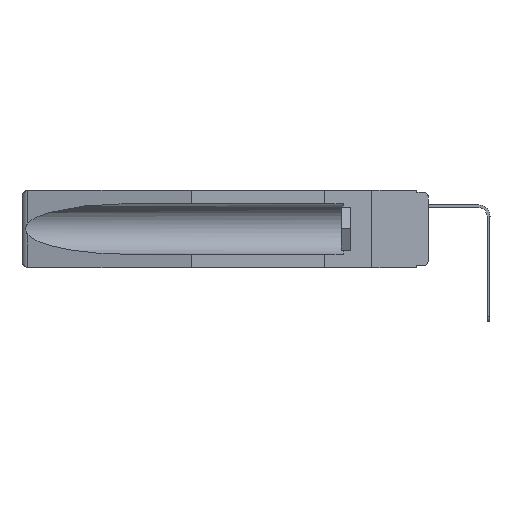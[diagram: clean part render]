
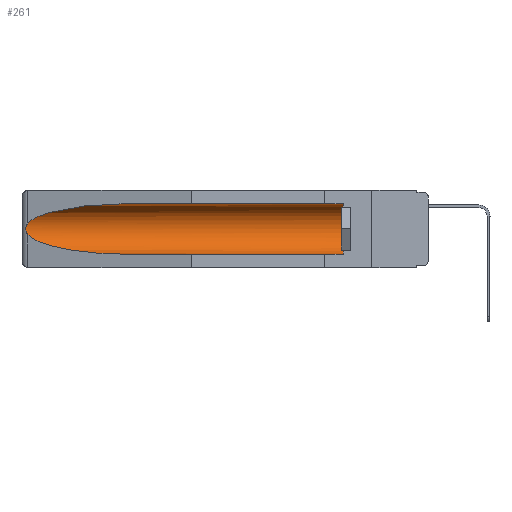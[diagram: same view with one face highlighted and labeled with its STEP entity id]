
A CAD part, left-side view. The second image highlights one B-rep face of the part: STEP entity #261.
In plain terms, the highlighted cylindrical face has radius 2.857 mm (diameter 5.715 mm), a partial arc.
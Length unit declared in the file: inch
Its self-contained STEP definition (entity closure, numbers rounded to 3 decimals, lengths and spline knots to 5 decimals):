
#261 = ADVANCED_FACE ( 'NONE', ( #9949 ), #20373, .F. ) ;
#1026 = DIRECTION ( 'NONE',  ( 0., 1., 0. ) ) ;
#1348 = EDGE_CURVE ( 'NONE', #8231, #16953, #18255, .T. ) ;
#1797 = ORIENTED_EDGE ( 'NONE', *, *, #7680, .F. ) ;
#2048 = CARTESIAN_POINT ( 'NONE',  ( 0.2673, 1.53269, -0.17917 ) ) ;
#2717 = CARTESIAN_POINT ( 'NONE',  ( 0.155, -0.30754, -0.059 ) ) ;
#2866 = DIRECTION ( 'NONE',  ( 0., -1., 0. ) ) ;
#4016 = DIRECTION ( 'NONE',  ( 0., 1., 0. ) ) ;
#4052 = VECTOR ( 'NONE', #4016, 39.37008 ) ;
#4215 = CARTESIAN_POINT ( 'NONE',  ( 0.21114, 1.30732, -0.059 ) ) ;
#4365 = CARTESIAN_POINT ( 'NONE',  ( 0.155, -0.30754, -0.1715 ) ) ;
#4412 = VECTOR ( 'NONE', #20978, 39.37008 ) ;
#4513 = DIRECTION ( 'NONE',  ( 0., 0., 1. ) ) ;
#5088 =( BOUNDED_CURVE ( )  B_SPLINE_CURVE ( 3, ( #14049, #4215, #5891, #16019 ),
 .UNSPECIFIED., .F., .T. ) 
 B_SPLINE_CURVE_WITH_KNOTS ( ( 4, 4 ),
 ( 4.71239, 6.08839 ),
 .UNSPECIFIED. ) 
 CURVE ( )  GEOMETRIC_REPRESENTATION_ITEM ( )  RATIONAL_B_SPLINE_CURVE ( ( 1., 0.848, 0.848, 1. ) ) 
 REPRESENTATION_ITEM ( '' )  );
#5197 = AXIS2_PLACEMENT_3D ( 'NONE', #4365, #1026, #14194 ) ;
#5366 = CARTESIAN_POINT ( 'NONE',  ( 0.26654, 1.53092, -0.15636 ) ) ;
#5609 = EDGE_LOOP ( 'NONE', ( #21602, #20404, #14075, #1797, #11931, #19507 ) ) ;
#5735 = EDGE_CURVE ( 'NONE', #16953, #8511, #5088, .T. ) ;
#5739 = CIRCLE ( 'NONE', #12850, 0.1125 ) ;
#5891 = CARTESIAN_POINT ( 'NONE',  ( 0.25451, 1.48313, -0.09465 ) ) ;
#6715 = CARTESIAN_POINT ( 'NONE',  ( 0.155, 0.126, -0.059 ) ) ;
#6747 = CARTESIAN_POINT ( 'NONE',  ( 0.26655, 1.53094, -0.18657 ) ) ;
#7036 = CARTESIAN_POINT ( 'NONE',  ( 0.2675, 1.53308, -0.16763 ) ) ;
#7680 = EDGE_CURVE ( 'NONE', #8990, #16061, #11639, .T. ) ;
#8231 = VERTEX_POINT ( 'NONE', #6715 ) ;
#8350 = CARTESIAN_POINT ( 'NONE',  ( 0.155, 1.07973, -0.059 ) ) ;
#8511 = VERTEX_POINT ( 'NONE', #13926 ) ;
#8990 = VERTEX_POINT ( 'NONE', #18480 ) ;
#9949 = FACE_OUTER_BOUND ( 'NONE', #5609, .T. ) ;
#10250 = CARTESIAN_POINT ( 'NONE',  ( 0.26597, 1.52961, -0.15275 ) ) ;
#10325 = CARTESIAN_POINT ( 'NONE',  ( 0.26537, 1.52718, -0.14972 ) ) ;
#10452 = CARTESIAN_POINT ( 'NONE',  ( 0.155, 1.07973, -0.284 ) ) ;
#10536 = CARTESIAN_POINT ( 'NONE',  ( 0.25451, 1.48313, -0.24835 ) ) ;
#10671 = CARTESIAN_POINT ( 'NONE',  ( 0.155, -0.30754, -0.284 ) ) ;
#11226 = CARTESIAN_POINT ( 'NONE',  ( 0.155, 0.126, -0.1715 ) ) ;
#11639 = LINE ( 'NONE', #10671, #4052 ) ;
#11931 = ORIENTED_EDGE ( 'NONE', *, *, #16201, .T. ) ;
#12039 = CARTESIAN_POINT ( 'NONE',  ( 0.26537, 1.52718, -0.19328 ) ) ;
#12171 = B_SPLINE_CURVE_WITH_KNOTS ( 'NONE', 3,
 ( #10325, #10250, #5366, #17023, #7036, #18706, #2048, #6747, #18424, #20079 ),
 .UNSPECIFIED., .F., .F.,
 ( 4, 2, 2, 2, 4 ),
 ( 0., 0.00029, 0.00058, 0.00087, 0.00117 ),
 .UNSPECIFIED. ) ;
#12664 = CARTESIAN_POINT ( 'NONE',  ( 0.26537, 1.52718, -0.19328 ) ) ;
#12850 = AXIS2_PLACEMENT_3D ( 'NONE', #11226, #2866, #4513 ) ;
#13782 = EDGE_CURVE ( 'NONE', #8511, #17865, #12171, .T. ) ;
#13926 = CARTESIAN_POINT ( 'NONE',  ( 0.26537, 1.52718, -0.14972 ) ) ;
#14049 = CARTESIAN_POINT ( 'NONE',  ( 0.155, 1.07973, -0.059 ) ) ;
#14075 = ORIENTED_EDGE ( 'NONE', *, *, #18277, .T. ) ;
#14194 = DIRECTION ( 'NONE',  ( 0., 0., 1. ) ) ;
#15263 = CARTESIAN_POINT ( 'NONE',  ( 0.21114, 1.30732, -0.284 ) ) ;
#16019 = CARTESIAN_POINT ( 'NONE',  ( 0.26537, 1.52718, -0.14972 ) ) ;
#16061 = VERTEX_POINT ( 'NONE', #17633 ) ;
#16201 = EDGE_CURVE ( 'NONE', #8990, #8231, #5739, .T. ) ;
#16711 =( BOUNDED_CURVE ( )  B_SPLINE_CURVE ( 3, ( #12039, #10536, #15263, #10452 ),
 .UNSPECIFIED., .F., .F. ) 
 B_SPLINE_CURVE_WITH_KNOTS ( ( 4, 4 ),
 ( 0.1948, 1.5708 ),
 .UNSPECIFIED. ) 
 CURVE ( )  GEOMETRIC_REPRESENTATION_ITEM ( )  RATIONAL_B_SPLINE_CURVE ( ( 1., 0.848, 0.848, 1. ) ) 
 REPRESENTATION_ITEM ( '' )  );
#16953 = VERTEX_POINT ( 'NONE', #8350 ) ;
#17023 = CARTESIAN_POINT ( 'NONE',  ( 0.2673, 1.5327, -0.16383 ) ) ;
#17633 = CARTESIAN_POINT ( 'NONE',  ( 0.155, 1.07973, -0.284 ) ) ;
#17865 = VERTEX_POINT ( 'NONE', #12664 ) ;
#18255 = LINE ( 'NONE', #2717, #4412 ) ;
#18277 = EDGE_CURVE ( 'NONE', #17865, #16061, #16711, .T. ) ;
#18424 = CARTESIAN_POINT ( 'NONE',  ( 0.26597, 1.5296, -0.19026 ) ) ;
#18480 = CARTESIAN_POINT ( 'NONE',  ( 0.155, 0.126, -0.284 ) ) ;
#18706 = CARTESIAN_POINT ( 'NONE',  ( 0.2675, 1.53308, -0.17534 ) ) ;
#19507 = ORIENTED_EDGE ( 'NONE', *, *, #1348, .T. ) ;
#20079 = CARTESIAN_POINT ( 'NONE',  ( 0.26537, 1.52718, -0.19328 ) ) ;
#20373 = CYLINDRICAL_SURFACE ( 'NONE', #5197, 0.1125 ) ;
#20404 = ORIENTED_EDGE ( 'NONE', *, *, #13782, .T. ) ;
#20978 = DIRECTION ( 'NONE',  ( 0., 1., 0. ) ) ;
#21602 = ORIENTED_EDGE ( 'NONE', *, *, #5735, .T. ) ;
